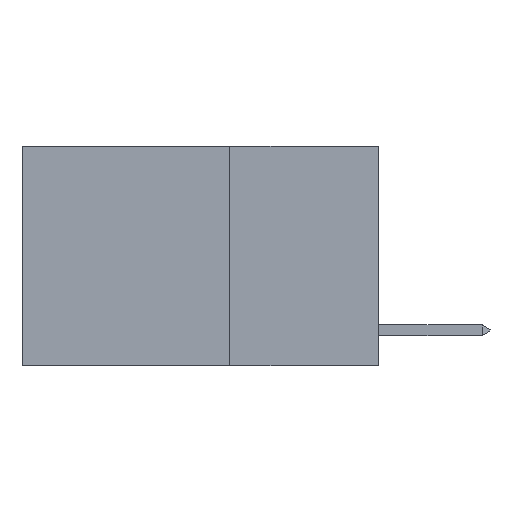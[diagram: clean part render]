
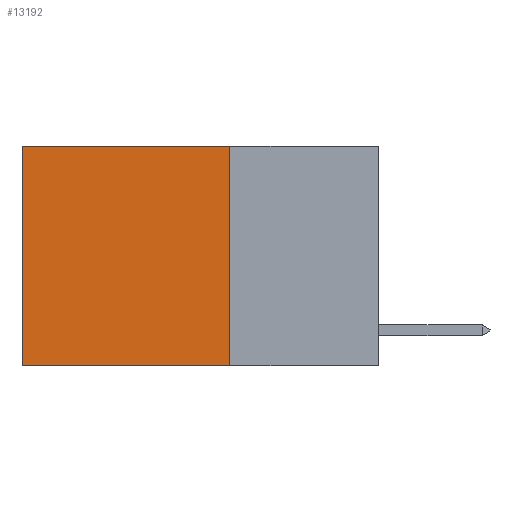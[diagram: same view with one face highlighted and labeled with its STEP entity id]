
A CAD part, left-side view. The second image highlights one B-rep face of the part: STEP entity #13192.
In plain terms, the highlighted planar face has unit normal (-1, 0, 0).
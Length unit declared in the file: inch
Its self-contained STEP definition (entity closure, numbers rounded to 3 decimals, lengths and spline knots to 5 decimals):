
#1770 = ORIENTED_EDGE ( 'NONE', *, *, #6844, .T. ) ;
#2479 = ORIENTED_EDGE ( 'NONE', *, *, #16935, .F. ) ;
#2840 = EDGE_LOOP ( 'NONE', ( #4834, #18938, #2479, #1770 ) ) ;
#3183 = EDGE_CURVE ( 'NONE', #20977, #12203, #15637, .T. ) ;
#3817 = DIRECTION ( 'NONE',  ( 1., 0., 0. ) ) ;
#4366 = FACE_OUTER_BOUND ( 'NONE', #2840, .T. ) ;
#4571 = VECTOR ( 'NONE', #11686, 39.37008 ) ;
#4834 = ORIENTED_EDGE ( 'NONE', *, *, #14332, .T. ) ;
#4974 = CARTESIAN_POINT ( 'NONE',  ( 0.2625, 0.6, 0. ) ) ;
#5223 = LINE ( 'NONE', #7261, #4571 ) ;
#6106 = DIRECTION ( 'NONE',  ( 0., 0., -1. ) ) ;
#6844 = EDGE_CURVE ( 'NONE', #23548, #22634, #5223, .T. ) ;
#7261 = CARTESIAN_POINT ( 'NONE',  ( 0.2625, 0.25, 0. ) ) ;
#7966 = CARTESIAN_POINT ( 'NONE',  ( 0.2625, 0.25, 0. ) ) ;
#8497 = CARTESIAN_POINT ( 'NONE',  ( 0.2625, 0.25, -0.37 ) ) ;
#10581 = CARTESIAN_POINT ( 'NONE',  ( 0.2625, 0.25, -0.37 ) ) ;
#11686 = DIRECTION ( 'NONE',  ( 0., 1., 0. ) ) ;
#12203 = VERTEX_POINT ( 'NONE', #26914 ) ;
#13192 = ADVANCED_FACE ( 'NONE', ( #4366 ), #24781, .F. ) ;
#14332 = EDGE_CURVE ( 'NONE', #22634, #12203, #14414, .T. ) ;
#14414 = LINE ( 'NONE', #15434, #24168 ) ;
#15317 = VECTOR ( 'NONE', #22878, 39.37008 ) ;
#15434 = CARTESIAN_POINT ( 'NONE',  ( 0.2625, 0.6, 0. ) ) ;
#15637 = LINE ( 'NONE', #8497, #15317 ) ;
#16935 = EDGE_CURVE ( 'NONE', #23548, #20977, #21693, .T. ) ;
#17640 = DIRECTION ( 'NONE',  ( 0., 0., -1. ) ) ;
#17851 = CARTESIAN_POINT ( 'NONE',  ( 0.2625, 0.25, 0. ) ) ;
#18585 = CARTESIAN_POINT ( 'NONE',  ( 0.2625, 0.25, 0. ) ) ;
#18938 = ORIENTED_EDGE ( 'NONE', *, *, #3183, .F. ) ;
#19960 = DIRECTION ( 'NONE',  ( 0., 0., -1. ) ) ;
#20977 = VERTEX_POINT ( 'NONE', #10581 ) ;
#21693 = LINE ( 'NONE', #17851, #23359 ) ;
#22634 = VERTEX_POINT ( 'NONE', #4974 ) ;
#22812 = AXIS2_PLACEMENT_3D ( 'NONE', #18585, #3817, #6106 ) ;
#22878 = DIRECTION ( 'NONE',  ( 0., 1., 0. ) ) ;
#23359 = VECTOR ( 'NONE', #19960, 39.37008 ) ;
#23548 = VERTEX_POINT ( 'NONE', #7966 ) ;
#24168 = VECTOR ( 'NONE', #17640, 39.37008 ) ;
#24781 = PLANE ( 'NONE',  #22812 ) ;
#26914 = CARTESIAN_POINT ( 'NONE',  ( 0.2625, 0.6, -0.37 ) ) ;
